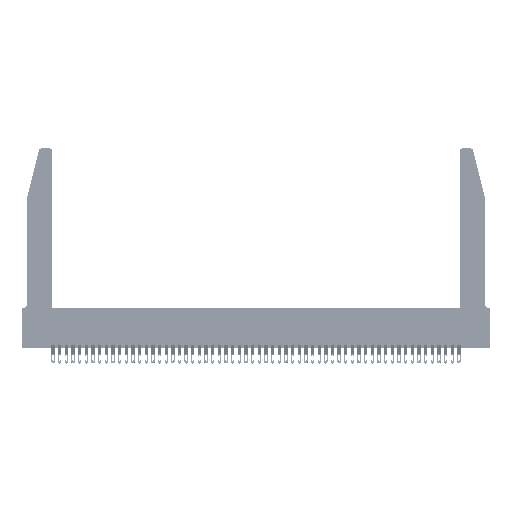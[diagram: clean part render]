
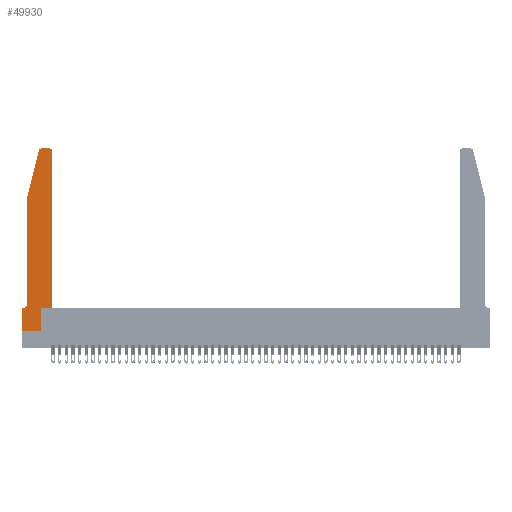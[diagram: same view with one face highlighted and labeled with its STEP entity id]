
A CAD part, top view. The second image highlights one B-rep face of the part: STEP entity #49930.
In plain terms, the highlighted planar face has unit normal (0, 0, 1).
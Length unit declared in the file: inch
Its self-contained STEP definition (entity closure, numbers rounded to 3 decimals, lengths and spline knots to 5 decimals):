
#62 = ORIENTED_EDGE ( 'NONE', *, *, #12183, .T. ) ;
#291 = DIRECTION ( 'NONE',  ( 0., 1., 0. ) ) ;
#496 = DIRECTION ( 'NONE',  ( 1., 0., 0. ) ) ;
#1040 = CARTESIAN_POINT ( 'NONE',  ( 0., 0., 0.37 ) ) ;
#1943 = CARTESIAN_POINT ( 'NONE',  ( 0.0755, 2., 0.37 ) ) ;
#2655 = ORIENTED_EDGE ( 'NONE', *, *, #30108, .T. ) ;
#3549 = DIRECTION ( 'NONE',  ( 1., 0., 0. ) ) ;
#4144 = ORIENTED_EDGE ( 'NONE', *, *, #26728, .T. ) ;
#4258 = VERTEX_POINT ( 'NONE', #7854 ) ;
#5125 = ORIENTED_EDGE ( 'NONE', *, *, #43399, .T. ) ;
#5525 = VERTEX_POINT ( 'NONE', #10405 ) ;
#6286 = AXIS2_PLACEMENT_3D ( 'NONE', #33269, #37392, #13840 ) ;
#6409 = DIRECTION ( 'NONE',  ( 1., 0., 0. ) ) ;
#7173 = CARTESIAN_POINT ( 'NONE',  ( 0.2865, 0.35, 0.37 ) ) ;
#7854 = CARTESIAN_POINT ( 'NONE',  ( 0., 0.35, 0.37 ) ) ;
#7965 = VECTOR ( 'NONE', #23993, 39.37008 ) ;
#8236 = ORIENTED_EDGE ( 'NONE', *, *, #37778, .T. ) ;
#8649 = EDGE_CURVE ( 'NONE', #37766, #17100, #21378, .T. ) ;
#10405 = CARTESIAN_POINT ( 'NONE',  ( 0.0055, 0.35, 0.37 ) ) ;
#10510 = CARTESIAN_POINT ( 'NONE',  ( 0.4505, 0.35, 0.37 ) ) ;
#10524 = EDGE_CURVE ( 'NONE', #4258, #27572, #45592, .T. ) ;
#10826 = AXIS2_PLACEMENT_3D ( 'NONE', #47942, #40325, #16765 ) ;
#11024 = VECTOR ( 'NONE', #18380, 39.37008 ) ;
#11163 = VERTEX_POINT ( 'NONE', #33660 ) ;
#11526 = CIRCLE ( 'NONE', #6286, 0.03 ) ;
#11642 = CARTESIAN_POINT ( 'NONE',  ( 0.4205, 2.72, 0.37 ) ) ;
#12028 = CARTESIAN_POINT ( 'NONE',  ( 0.25487, 2.72718, 0.37 ) ) ;
#12183 = EDGE_CURVE ( 'NONE', #27572, #39082, #13977, .T. ) ;
#12322 = FACE_OUTER_BOUND ( 'NONE', #42844, .T. ) ;
#12409 = LINE ( 'NONE', #1943, #35813 ) ;
#13840 = DIRECTION ( 'NONE',  ( 1., 0., 0. ) ) ;
#13954 = ORIENTED_EDGE ( 'NONE', *, *, #46841, .T. ) ;
#13977 = LINE ( 'NONE', #1040, #29993 ) ;
#14215 = CIRCLE ( 'NONE', #10826, 0.07 ) ;
#14250 = VERTEX_POINT ( 'NONE', #40206 ) ;
#14676 = VERTEX_POINT ( 'NONE', #31068 ) ;
#15123 = CIRCLE ( 'NONE', #41553, 0.03 ) ;
#16220 = VECTOR ( 'NONE', #28424, 39.37008 ) ;
#16377 = LINE ( 'NONE', #28227, #23151 ) ;
#16748 = EDGE_CURVE ( 'NONE', #14250, #24845, #42525, .T. ) ;
#16765 = DIRECTION ( 'NONE',  ( -1., 0., 0. ) ) ;
#17100 = VERTEX_POINT ( 'NONE', #10510 ) ;
#17464 = LINE ( 'NONE', #44049, #16220 ) ;
#18380 = DIRECTION ( 'NONE',  ( -1., 0., 0. ) ) ;
#18889 = CARTESIAN_POINT ( 'NONE',  ( 0.0755, 2., 0.37 ) ) ;
#19079 = ORIENTED_EDGE ( 'NONE', *, *, #19738, .T. ) ;
#19405 = CARTESIAN_POINT ( 'NONE',  ( 0., 0., 0.37 ) ) ;
#19738 = EDGE_CURVE ( 'NONE', #39082, #37766, #16377, .T. ) ;
#21378 = LINE ( 'NONE', #36714, #48490 ) ;
#22454 = CARTESIAN_POINT ( 'NONE',  ( 0., 0.35, 0.37 ) ) ;
#23151 = VECTOR ( 'NONE', #291, 39.37008 ) ;
#23688 = DIRECTION ( 'NONE',  ( 0., 0., 1. ) ) ;
#23993 = DIRECTION ( 'NONE',  ( 0., -1., 0. ) ) ;
#24617 = ORIENTED_EDGE ( 'NONE', *, *, #42193, .T. ) ;
#24845 = VERTEX_POINT ( 'NONE', #35899 ) ;
#25919 = DIRECTION ( 'NONE',  ( -0.239, -0.971, 0. ) ) ;
#26728 = EDGE_CURVE ( 'NONE', #14676, #5525, #14215, .T. ) ;
#27572 = VERTEX_POINT ( 'NONE', #19405 ) ;
#27802 = VECTOR ( 'NONE', #27890, 39.37008 ) ;
#27890 = DIRECTION ( 'NONE',  ( -1., 0., 0. ) ) ;
#28227 = CARTESIAN_POINT ( 'NONE',  ( 0.2865, 0.35, 0.37 ) ) ;
#28303 = AXIS2_PLACEMENT_3D ( 'NONE', #22454, #50525, #50357 ) ;
#28306 = CARTESIAN_POINT ( 'NONE',  ( 0., 0., 0.37 ) ) ;
#28424 = DIRECTION ( 'NONE',  ( 0., 1., 0. ) ) ;
#29993 = VECTOR ( 'NONE', #496, 39.37008 ) ;
#30108 = EDGE_CURVE ( 'NONE', #24845, #41576, #11526, .T. ) ;
#31068 = CARTESIAN_POINT ( 'NONE',  ( 0.0755, 0.42, 0.37 ) ) ;
#31115 = DIRECTION ( 'NONE',  ( 0., -1., 0. ) ) ;
#33071 = EDGE_CURVE ( 'NONE', #41576, #39427, #12409, .T. ) ;
#33269 = CARTESIAN_POINT ( 'NONE',  ( 0.284, 2.72, 0.37 ) ) ;
#33660 = CARTESIAN_POINT ( 'NONE',  ( 0.4505, 2.72, 0.37 ) ) ;
#33874 = CARTESIAN_POINT ( 'NONE',  ( 0.0755, 0.35, 0.37 ) ) ;
#34514 = VECTOR ( 'NONE', #31115, 39.37008 ) ;
#35813 = VECTOR ( 'NONE', #25919, 39.37008 ) ;
#35899 = CARTESIAN_POINT ( 'NONE',  ( 0.284, 2.75, 0.37 ) ) ;
#36714 = CARTESIAN_POINT ( 'NONE',  ( 0.4505, 0.35, 0.37 ) ) ;
#37392 = DIRECTION ( 'NONE',  ( 0., 0., 1. ) ) ;
#37766 = VERTEX_POINT ( 'NONE', #7173 ) ;
#37778 = EDGE_CURVE ( 'NONE', #39427, #14676, #38802, .T. ) ;
#38802 = LINE ( 'NONE', #18889, #34514 ) ;
#39082 = VERTEX_POINT ( 'NONE', #46509 ) ;
#39427 = VERTEX_POINT ( 'NONE', #47699 ) ;
#40072 = CARTESIAN_POINT ( 'NONE',  ( 0.2605, 2.75, 0.37 ) ) ;
#40206 = CARTESIAN_POINT ( 'NONE',  ( 0.4205, 2.75, 0.37 ) ) ;
#40296 = ORIENTED_EDGE ( 'NONE', *, *, #33071, .T. ) ;
#40325 = DIRECTION ( 'NONE',  ( 0., 0., -1. ) ) ;
#41553 = AXIS2_PLACEMENT_3D ( 'NONE', #11642, #23688, #3549 ) ;
#41576 = VERTEX_POINT ( 'NONE', #12028 ) ;
#42193 = EDGE_CURVE ( 'NONE', #11163, #14250, #15123, .T. ) ;
#42525 = LINE ( 'NONE', #40072, #27802 ) ;
#42844 = EDGE_LOOP ( 'NONE', ( #43568, #2655, #40296, #8236, #4144, #13954, #45732, #62, #19079, #47436, #5125, #24617 ) ) ;
#43399 = EDGE_CURVE ( 'NONE', #17100, #11163, #17464, .T. ) ;
#43568 = ORIENTED_EDGE ( 'NONE', *, *, #16748, .T. ) ;
#44049 = CARTESIAN_POINT ( 'NONE',  ( 0.4505, 0.35, 0.37 ) ) ;
#44251 = LINE ( 'NONE', #33874, #11024 ) ;
#45592 = LINE ( 'NONE', #28306, #7965 ) ;
#45732 = ORIENTED_EDGE ( 'NONE', *, *, #10524, .T. ) ;
#46509 = CARTESIAN_POINT ( 'NONE',  ( 0.2865, 0., 0.37 ) ) ;
#46841 = EDGE_CURVE ( 'NONE', #5525, #4258, #44251, .T. ) ;
#47436 = ORIENTED_EDGE ( 'NONE', *, *, #8649, .T. ) ;
#47699 = CARTESIAN_POINT ( 'NONE',  ( 0.0755, 2., 0.37 ) ) ;
#47942 = CARTESIAN_POINT ( 'NONE',  ( 0.0055, 0.42, 0.37 ) ) ;
#48490 = VECTOR ( 'NONE', #6409, 39.37008 ) ;
#49850 = PLANE ( 'NONE',  #28303 ) ;
#49930 = ADVANCED_FACE ( 'NONE', ( #12322 ), #49850, .T. ) ;
#50357 = DIRECTION ( 'NONE',  ( 1., 0., 0. ) ) ;
#50525 = DIRECTION ( 'NONE',  ( 0., 0., 1. ) ) ;
